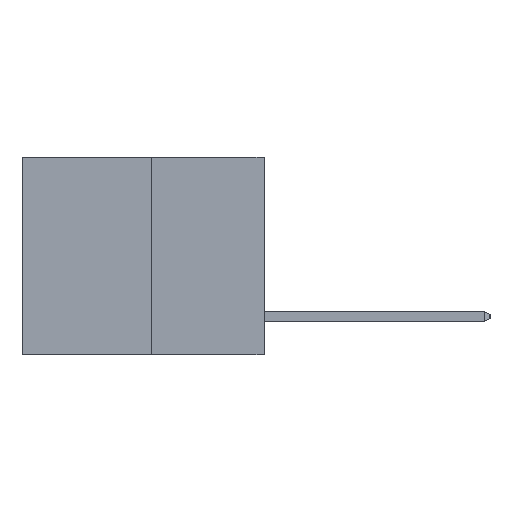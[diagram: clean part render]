
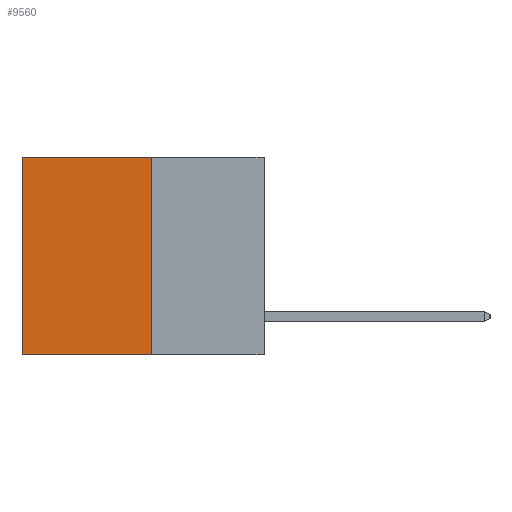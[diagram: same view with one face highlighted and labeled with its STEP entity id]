
A CAD part, left-side view. The second image highlights one B-rep face of the part: STEP entity #9560.
In plain terms, the highlighted planar face has unit normal (-1, 0, 0).
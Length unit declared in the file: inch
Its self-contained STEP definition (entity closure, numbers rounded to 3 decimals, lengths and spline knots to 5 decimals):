
#146 = VECTOR ( 'NONE', #4622, 39.37008 ) ;
#515 = LINE ( 'NONE', #8689, #11389 ) ;
#536 = DIRECTION ( 'NONE',  ( 0., 1., 0. ) ) ;
#740 = CARTESIAN_POINT ( 'NONE',  ( 0.3165, 0.6, -0.49 ) ) ;
#864 = CARTESIAN_POINT ( 'NONE',  ( 0.3165, 0.28, -0.49 ) ) ;
#1253 = VECTOR ( 'NONE', #7184, 39.37008 ) ;
#1741 = EDGE_CURVE ( 'NONE', #4755, #2005, #9182, .T. ) ;
#1878 = ORIENTED_EDGE ( 'NONE', *, *, #10189, .T. ) ;
#2005 = VERTEX_POINT ( 'NONE', #3227 ) ;
#2089 = LINE ( 'NONE', #740, #1253 ) ;
#2899 = EDGE_LOOP ( 'NONE', ( #7089, #7551, #10083, #1878 ) ) ;
#3227 = CARTESIAN_POINT ( 'NONE',  ( 0.3165, 0.6, -0.49 ) ) ;
#3333 = CARTESIAN_POINT ( 'NONE',  ( 0.3165, 0.6, 0. ) ) ;
#3905 = LINE ( 'NONE', #5691, #11328 ) ;
#4622 = DIRECTION ( 'NONE',  ( 0., 1., 0. ) ) ;
#4755 = VERTEX_POINT ( 'NONE', #864 ) ;
#5447 = DIRECTION ( 'NONE',  ( 0., 0., -1. ) ) ;
#5691 = CARTESIAN_POINT ( 'NONE',  ( 0.3165, 0.28, 0. ) ) ;
#6235 = CARTESIAN_POINT ( 'NONE',  ( 0.3165, 0.28, -0.49 ) ) ;
#6628 = CARTESIAN_POINT ( 'NONE',  ( 0.3165, 0.28, 0. ) ) ;
#7089 = ORIENTED_EDGE ( 'NONE', *, *, #11264, .T. ) ;
#7184 = DIRECTION ( 'NONE',  ( 0., 0., -1. ) ) ;
#7551 = ORIENTED_EDGE ( 'NONE', *, *, #1741, .F. ) ;
#7657 = CARTESIAN_POINT ( 'NONE',  ( 0.3165, 0.28, -0.49 ) ) ;
#8245 = EDGE_CURVE ( 'NONE', #12162, #4755, #515, .T. ) ;
#8689 = CARTESIAN_POINT ( 'NONE',  ( 0.3165, 0.28, -0.49 ) ) ;
#9182 = LINE ( 'NONE', #7657, #146 ) ;
#9293 = DIRECTION ( 'NONE',  ( 1., 0., 0. ) ) ;
#9560 = ADVANCED_FACE ( 'NONE', ( #10868 ), #13509, .F. ) ;
#10083 = ORIENTED_EDGE ( 'NONE', *, *, #8245, .F. ) ;
#10189 = EDGE_CURVE ( 'NONE', #12162, #11422, #3905, .T. ) ;
#10267 = AXIS2_PLACEMENT_3D ( 'NONE', #6235, #9293, #10454 ) ;
#10454 = DIRECTION ( 'NONE',  ( 0., 0., -1. ) ) ;
#10868 = FACE_OUTER_BOUND ( 'NONE', #2899, .T. ) ;
#11264 = EDGE_CURVE ( 'NONE', #11422, #2005, #2089, .T. ) ;
#11328 = VECTOR ( 'NONE', #536, 39.37008 ) ;
#11389 = VECTOR ( 'NONE', #5447, 39.37008 ) ;
#11422 = VERTEX_POINT ( 'NONE', #3333 ) ;
#12162 = VERTEX_POINT ( 'NONE', #6628 ) ;
#13509 = PLANE ( 'NONE',  #10267 ) ;
